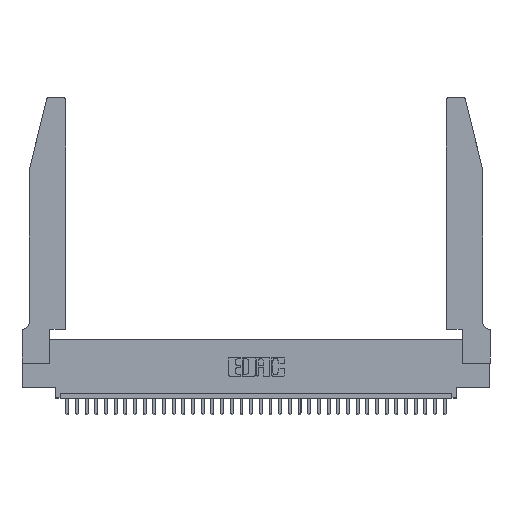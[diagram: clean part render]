
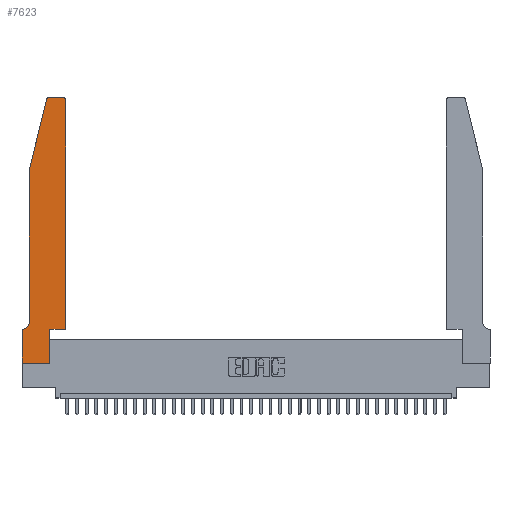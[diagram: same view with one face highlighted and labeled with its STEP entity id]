
A CAD part, top view. The second image highlights one B-rep face of the part: STEP entity #7623.
In plain terms, the highlighted planar face has unit normal (0, 0, 1).
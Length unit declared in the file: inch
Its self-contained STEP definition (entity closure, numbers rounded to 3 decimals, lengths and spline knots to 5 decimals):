
#41 = CARTESIAN_POINT ( 'NONE',  ( 0.4505, 0.35, 0.37 ) ) ;
#138 = CARTESIAN_POINT ( 'NONE',  ( 0.284, 2.72, 0.37 ) ) ;
#195 = CARTESIAN_POINT ( 'NONE',  ( 0., 0., 0.37 ) ) ;
#315 = EDGE_CURVE ( 'NONE', #15561, #17732, #17904, .T. ) ;
#793 = VERTEX_POINT ( 'NONE', #18059 ) ;
#1080 = ORIENTED_EDGE ( 'NONE', *, *, #32745, .T. ) ;
#1654 = LINE ( 'NONE', #31120, #29740 ) ;
#1702 = CIRCLE ( 'NONE', #32480, 0.07 ) ;
#2328 = PLANE ( 'NONE',  #26554 ) ;
#2601 = DIRECTION ( 'NONE',  ( 0., 0., -1. ) ) ;
#2630 = DIRECTION ( 'NONE',  ( 1., 0., 0. ) ) ;
#2645 = LINE ( 'NONE', #24866, #11594 ) ;
#2707 = CIRCLE ( 'NONE', #29690, 0.03 ) ;
#2760 = EDGE_CURVE ( 'NONE', #28765, #6298, #20751, .T. ) ;
#3059 = CARTESIAN_POINT ( 'NONE',  ( 0.0755, 0.35, 0.37 ) ) ;
#3113 = CARTESIAN_POINT ( 'NONE',  ( 0.25487, 2.72718, 0.37 ) ) ;
#3183 = DIRECTION ( 'NONE',  ( -1., 0., 0. ) ) ;
#3301 = ORIENTED_EDGE ( 'NONE', *, *, #23819, .T. ) ;
#3456 = ORIENTED_EDGE ( 'NONE', *, *, #17771, .T. ) ;
#3821 = EDGE_CURVE ( 'NONE', #5922, #28765, #24881, .T. ) ;
#4178 = ORIENTED_EDGE ( 'NONE', *, *, #34965, .T. ) ;
#4807 = AXIS2_PLACEMENT_3D ( 'NONE', #138, #13570, #16284 ) ;
#5831 = DIRECTION ( 'NONE',  ( 1., 0., 0. ) ) ;
#5922 = VERTEX_POINT ( 'NONE', #11073 ) ;
#6298 = VERTEX_POINT ( 'NONE', #7090 ) ;
#7090 = CARTESIAN_POINT ( 'NONE',  ( 0.4505, 0.35, 0.37 ) ) ;
#7623 = ADVANCED_FACE ( 'NONE', ( #15627 ), #2328, .T. ) ;
#7630 = CARTESIAN_POINT ( 'NONE',  ( 0.284, 2.75, 0.37 ) ) ;
#9260 = DIRECTION ( 'NONE',  ( -0.239, -0.971, 0. ) ) ;
#9283 = VECTOR ( 'NONE', #15417, 39.37008 ) ;
#9476 = VERTEX_POINT ( 'NONE', #7630 ) ;
#10435 = VECTOR ( 'NONE', #3183, 39.37008 ) ;
#10573 = CARTESIAN_POINT ( 'NONE',  ( 0., 0., 0.37 ) ) ;
#10659 = VERTEX_POINT ( 'NONE', #3113 ) ;
#11073 = CARTESIAN_POINT ( 'NONE',  ( 0.2865, 0., 0.37 ) ) ;
#11594 = VECTOR ( 'NONE', #16711, 39.37008 ) ;
#12408 = CARTESIAN_POINT ( 'NONE',  ( 0.4205, 2.75, 0.37 ) ) ;
#13488 = LINE ( 'NONE', #17087, #26291 ) ;
#13506 = EDGE_CURVE ( 'NONE', #30161, #9476, #13488, .T. ) ;
#13540 = DIRECTION ( 'NONE',  ( -1., 0., 0. ) ) ;
#13543 = VECTOR ( 'NONE', #29859, 39.37008 ) ;
#13570 = DIRECTION ( 'NONE',  ( 0., 0., 1. ) ) ;
#13767 = VERTEX_POINT ( 'NONE', #15976 ) ;
#14530 = CARTESIAN_POINT ( 'NONE',  ( 0.0055, 0.35, 0.37 ) ) ;
#15417 = DIRECTION ( 'NONE',  ( 0., -1., 0. ) ) ;
#15548 = VERTEX_POINT ( 'NONE', #14530 ) ;
#15561 = VERTEX_POINT ( 'NONE', #16881 ) ;
#15627 = FACE_OUTER_BOUND ( 'NONE', #16860, .T. ) ;
#15976 = CARTESIAN_POINT ( 'NONE',  ( 0.0755, 0.42, 0.37 ) ) ;
#16014 = VECTOR ( 'NONE', #21712, 39.37008 ) ;
#16284 = DIRECTION ( 'NONE',  ( 1., 0., 0. ) ) ;
#16610 = VECTOR ( 'NONE', #24056, 39.37008 ) ;
#16711 = DIRECTION ( 'NONE',  ( 0., 1., 0. ) ) ;
#16860 = EDGE_LOOP ( 'NONE', ( #21561, #31054, #20939, #1080, #4178, #22689, #24140, #17703, #26106, #32589, #3301, #3456 ) ) ;
#16881 = CARTESIAN_POINT ( 'NONE',  ( 0., 0.35, 0.37 ) ) ;
#17087 = CARTESIAN_POINT ( 'NONE',  ( 0.2605, 2.75, 0.37 ) ) ;
#17496 = EDGE_CURVE ( 'NONE', #9476, #10659, #19298, .T. ) ;
#17630 = CARTESIAN_POINT ( 'NONE',  ( 0., 0.35, 0.37 ) ) ;
#17663 = LINE ( 'NONE', #3059, #10435 ) ;
#17703 = ORIENTED_EDGE ( 'NONE', *, *, #34939, .T. ) ;
#17732 = VERTEX_POINT ( 'NONE', #195 ) ;
#17771 = EDGE_CURVE ( 'NONE', #21839, #30161, #2707, .T. ) ;
#17904 = LINE ( 'NONE', #10573, #16610 ) ;
#18059 = CARTESIAN_POINT ( 'NONE',  ( 0.0755, 2., 0.37 ) ) ;
#19050 = DIRECTION ( 'NONE',  ( 0., 0., 1. ) ) ;
#19298 = CIRCLE ( 'NONE', #4807, 0.03 ) ;
#20645 = CARTESIAN_POINT ( 'NONE',  ( 0.2865, 0.35, 0.37 ) ) ;
#20751 = LINE ( 'NONE', #41, #16014 ) ;
#20939 = ORIENTED_EDGE ( 'NONE', *, *, #32582, .T. ) ;
#21329 = CARTESIAN_POINT ( 'NONE',  ( 0.0055, 0.42, 0.37 ) ) ;
#21561 = ORIENTED_EDGE ( 'NONE', *, *, #13506, .T. ) ;
#21712 = DIRECTION ( 'NONE',  ( 1., 0., 0. ) ) ;
#21839 = VERTEX_POINT ( 'NONE', #25462 ) ;
#22689 = ORIENTED_EDGE ( 'NONE', *, *, #28849, .T. ) ;
#23436 = LINE ( 'NONE', #35088, #13543 ) ;
#23819 = EDGE_CURVE ( 'NONE', #6298, #21839, #2645, .T. ) ;
#24056 = DIRECTION ( 'NONE',  ( 0., -1., 0. ) ) ;
#24140 = ORIENTED_EDGE ( 'NONE', *, *, #315, .T. ) ;
#24866 = CARTESIAN_POINT ( 'NONE',  ( 0.4505, 0.35, 0.37 ) ) ;
#24881 = LINE ( 'NONE', #20645, #29951 ) ;
#25148 = CARTESIAN_POINT ( 'NONE',  ( 0.4205, 2.72, 0.37 ) ) ;
#25462 = CARTESIAN_POINT ( 'NONE',  ( 0.4505, 2.72, 0.37 ) ) ;
#26106 = ORIENTED_EDGE ( 'NONE', *, *, #3821, .T. ) ;
#26129 = DIRECTION ( 'NONE',  ( 0., 1., 0. ) ) ;
#26287 = CARTESIAN_POINT ( 'NONE',  ( 0.0755, 2., 0.37 ) ) ;
#26291 = VECTOR ( 'NONE', #33284, 39.37008 ) ;
#26554 = AXIS2_PLACEMENT_3D ( 'NONE', #17630, #19050, #2630 ) ;
#27852 = DIRECTION ( 'NONE',  ( 0., 0., 1. ) ) ;
#28765 = VERTEX_POINT ( 'NONE', #29748 ) ;
#28849 = EDGE_CURVE ( 'NONE', #15548, #15561, #17663, .T. ) ;
#29690 = AXIS2_PLACEMENT_3D ( 'NONE', #25148, #27852, #5831 ) ;
#29740 = VECTOR ( 'NONE', #9260, 39.37008 ) ;
#29748 = CARTESIAN_POINT ( 'NONE',  ( 0.2865, 0.35, 0.37 ) ) ;
#29859 = DIRECTION ( 'NONE',  ( 1., 0., 0. ) ) ;
#29951 = VECTOR ( 'NONE', #26129, 39.37008 ) ;
#30161 = VERTEX_POINT ( 'NONE', #12408 ) ;
#31054 = ORIENTED_EDGE ( 'NONE', *, *, #17496, .T. ) ;
#31120 = CARTESIAN_POINT ( 'NONE',  ( 0.0755, 2., 0.37 ) ) ;
#32480 = AXIS2_PLACEMENT_3D ( 'NONE', #21329, #2601, #13540 ) ;
#32582 = EDGE_CURVE ( 'NONE', #10659, #793, #1654, .T. ) ;
#32589 = ORIENTED_EDGE ( 'NONE', *, *, #2760, .T. ) ;
#32745 = EDGE_CURVE ( 'NONE', #793, #13767, #33222, .T. ) ;
#33222 = LINE ( 'NONE', #26287, #9283 ) ;
#33284 = DIRECTION ( 'NONE',  ( -1., 0., 0. ) ) ;
#34939 = EDGE_CURVE ( 'NONE', #17732, #5922, #23436, .T. ) ;
#34965 = EDGE_CURVE ( 'NONE', #13767, #15548, #1702, .T. ) ;
#35088 = CARTESIAN_POINT ( 'NONE',  ( 0., 0., 0.37 ) ) ;
